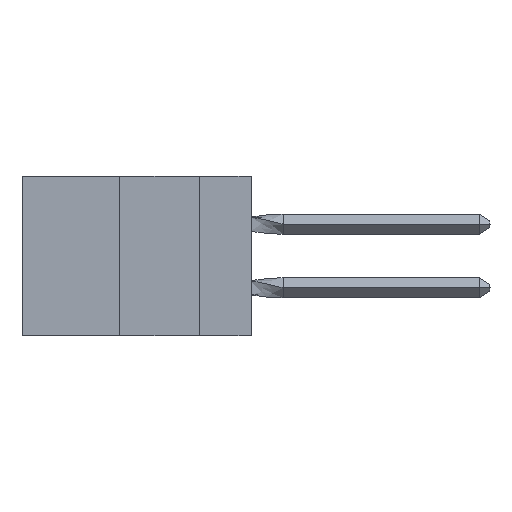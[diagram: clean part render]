
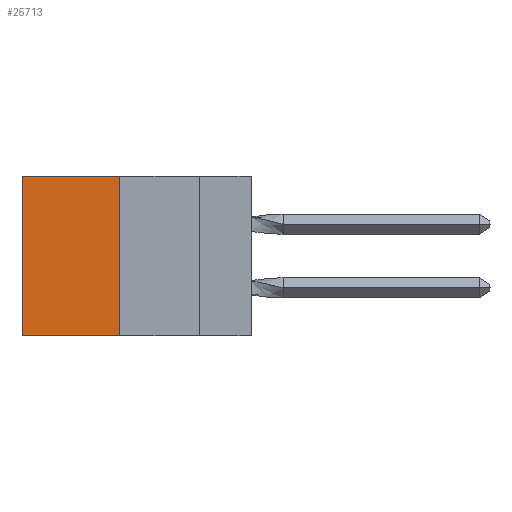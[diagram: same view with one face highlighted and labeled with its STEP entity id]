
A CAD part, left-side view. The second image highlights one B-rep face of the part: STEP entity #25713.
In plain terms, the highlighted planar face has unit normal (-1, 0, 0).
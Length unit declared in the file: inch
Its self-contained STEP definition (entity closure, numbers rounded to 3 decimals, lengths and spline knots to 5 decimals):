
#1178 = LINE ( 'NONE', #16498, #30033 ) ;
#2368 = LINE ( 'NONE', #22458, #24672 ) ;
#3560 = AXIS2_PLACEMENT_3D ( 'NONE', #6753, #15358, #29216 ) ;
#3656 = DIRECTION ( 'NONE',  ( 0., 1., 0. ) ) ;
#3932 = PLANE ( 'NONE',  #3560 ) ;
#4103 = EDGE_CURVE ( 'NONE', #27405, #4578, #2368, .T. ) ;
#4578 = VERTEX_POINT ( 'NONE', #36200 ) ;
#4999 = EDGE_CURVE ( 'NONE', #35202, #4578, #19000, .T. ) ;
#6753 = CARTESIAN_POINT ( 'NONE',  ( 0.305, 0.413, -0.5 ) ) ;
#13790 = CARTESIAN_POINT ( 'NONE',  ( 0.305, 0.413, -0.5 ) ) ;
#14251 = VECTOR ( 'NONE', #18197, 39.37008 ) ;
#14660 = FACE_OUTER_BOUND ( 'NONE', #34994, .T. ) ;
#15358 = DIRECTION ( 'NONE',  ( 1., 0., 0. ) ) ;
#16498 = CARTESIAN_POINT ( 'NONE',  ( 0.305, 0.413, -0.5 ) ) ;
#18197 = DIRECTION ( 'NONE',  ( 0., 0., -1. ) ) ;
#18686 = ORIENTED_EDGE ( 'NONE', *, *, #32776, .F. ) ;
#19000 = LINE ( 'NONE', #32087, #14251 ) ;
#20711 = EDGE_CURVE ( 'NONE', #24601, #35202, #29989, .T. ) ;
#22458 = CARTESIAN_POINT ( 'NONE',  ( 0.305, 0.413, -0.5 ) ) ;
#22870 = CARTESIAN_POINT ( 'NONE',  ( 0.305, 0.413, 0. ) ) ;
#24601 = VERTEX_POINT ( 'NONE', #28129 ) ;
#24672 = VECTOR ( 'NONE', #36117, 39.37008 ) ;
#25713 = ADVANCED_FACE ( 'NONE', ( #14660 ), #3932, .F. ) ;
#27405 = VERTEX_POINT ( 'NONE', #13790 ) ;
#27556 = DIRECTION ( 'NONE',  ( 0., 0., -1. ) ) ;
#28129 = CARTESIAN_POINT ( 'NONE',  ( 0.305, 0.413, 0. ) ) ;
#28320 = CARTESIAN_POINT ( 'NONE',  ( 0.305, 0.72, 0. ) ) ;
#28644 = VECTOR ( 'NONE', #3656, 39.37008 ) ;
#29216 = DIRECTION ( 'NONE',  ( 0., 0., -1. ) ) ;
#29989 = LINE ( 'NONE', #22870, #28644 ) ;
#30033 = VECTOR ( 'NONE', #27556, 39.37008 ) ;
#30048 = ORIENTED_EDGE ( 'NONE', *, *, #4103, .F. ) ;
#32087 = CARTESIAN_POINT ( 'NONE',  ( 0.305, 0.72, -0.5 ) ) ;
#32776 = EDGE_CURVE ( 'NONE', #24601, #27405, #1178, .T. ) ;
#32970 = ORIENTED_EDGE ( 'NONE', *, *, #20711, .T. ) ;
#34994 = EDGE_LOOP ( 'NONE', ( #35373, #30048, #18686, #32970 ) ) ;
#35202 = VERTEX_POINT ( 'NONE', #28320 ) ;
#35373 = ORIENTED_EDGE ( 'NONE', *, *, #4999, .T. ) ;
#36117 = DIRECTION ( 'NONE',  ( 0., 1., 0. ) ) ;
#36200 = CARTESIAN_POINT ( 'NONE',  ( 0.305, 0.72, -0.5 ) ) ;
